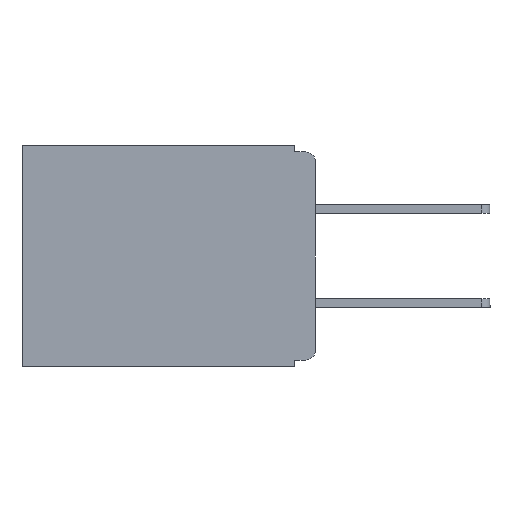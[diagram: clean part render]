
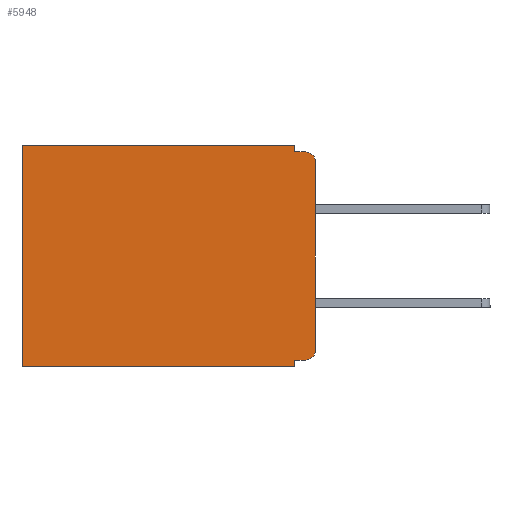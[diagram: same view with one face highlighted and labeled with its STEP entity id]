
A CAD part, left-side view. The second image highlights one B-rep face of the part: STEP entity #5948.
In plain terms, the highlighted planar face has unit normal (-1, 0, 0).
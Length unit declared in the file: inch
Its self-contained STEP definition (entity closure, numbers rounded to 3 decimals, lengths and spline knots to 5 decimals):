
#45 = DIRECTION ( 'NONE',  ( 0., 0., -1. ) ) ;
#48 = EDGE_CURVE ( 'NONE', #10251, #4668, #8956, .T. ) ;
#84 = ORIENTED_EDGE ( 'NONE', *, *, #4038, .F. ) ;
#166 = ORIENTED_EDGE ( 'NONE', *, *, #9254, .T. ) ;
#447 = CARTESIAN_POINT ( 'NONE',  ( 0.3, 0.437, 0. ) ) ;
#504 = AXIS2_PLACEMENT_3D ( 'NONE', #6257, #778, #7069 ) ;
#517 = FACE_OUTER_BOUND ( 'NONE', #5167, .T. ) ;
#527 = ORIENTED_EDGE ( 'NONE', *, *, #8979, .F. ) ;
#778 = DIRECTION ( 'NONE',  ( -1., 0., 0. ) ) ;
#1246 = DIRECTION ( 'NONE',  ( 0., 1., 0. ) ) ;
#1308 = VERTEX_POINT ( 'NONE', #2556 ) ;
#1347 = CARTESIAN_POINT ( 'NONE',  ( 0.3, 0.015, -0.32 ) ) ;
#1393 = EDGE_CURVE ( 'NONE', #7109, #4877, #10138, .T. ) ;
#1486 = ORIENTED_EDGE ( 'NONE', *, *, #9015, .T. ) ;
#1816 = CARTESIAN_POINT ( 'NONE',  ( 0.3, 0., 0. ) ) ;
#1908 = CIRCLE ( 'NONE', #504, 0.015 ) ;
#2293 = VECTOR ( 'NONE', #5901, 39.37008 ) ;
#2328 = VERTEX_POINT ( 'NONE', #2756 ) ;
#2369 = VECTOR ( 'NONE', #7701, 39.37008 ) ;
#2556 = CARTESIAN_POINT ( 'NONE',  ( 0.3, 0.031, 0. ) ) ;
#2640 = AXIS2_PLACEMENT_3D ( 'NONE', #8299, #3280, #9024 ) ;
#2756 = CARTESIAN_POINT ( 'NONE',  ( 0.3, 0., -0.305 ) ) ;
#2827 = CARTESIAN_POINT ( 'NONE',  ( 0.3, 0.031, -0.32 ) ) ;
#3158 = CARTESIAN_POINT ( 'NONE',  ( 0.3, 0.031, -0.01 ) ) ;
#3280 = DIRECTION ( 'NONE',  ( -1., 0., 0. ) ) ;
#3323 = ORIENTED_EDGE ( 'NONE', *, *, #4659, .F. ) ;
#3434 = VERTEX_POINT ( 'NONE', #7108 ) ;
#3582 = EDGE_CURVE ( 'NONE', #1308, #7109, #7062, .T. ) ;
#3742 = LINE ( 'NONE', #5969, #7959 ) ;
#3849 = VECTOR ( 'NONE', #45, 39.37008 ) ;
#4038 = EDGE_CURVE ( 'NONE', #4668, #4877, #8539, .T. ) ;
#4199 = VECTOR ( 'NONE', #10359, 39.37008 ) ;
#4332 = CARTESIAN_POINT ( 'NONE',  ( 0.3, 0., -0.33 ) ) ;
#4659 = EDGE_CURVE ( 'NONE', #1308, #5232, #3742, .T. ) ;
#4668 = VERTEX_POINT ( 'NONE', #5584 ) ;
#4790 = LINE ( 'NONE', #4332, #2369 ) ;
#4877 = VERTEX_POINT ( 'NONE', #5928 ) ;
#5167 = EDGE_LOOP ( 'NONE', ( #9774, #1486, #5932, #3323, #10086, #9341, #84, #9676, #527, #166 ) ) ;
#5197 = CARTESIAN_POINT ( 'NONE',  ( 0.3, 0.437, -0.33 ) ) ;
#5232 = VERTEX_POINT ( 'NONE', #3158 ) ;
#5358 = PLANE ( 'NONE',  #9312 ) ;
#5584 = CARTESIAN_POINT ( 'NONE',  ( 0.3, 0.031, -0.33 ) ) ;
#5602 = DIRECTION ( 'NONE',  ( 0., 0., -1. ) ) ;
#5901 = DIRECTION ( 'NONE',  ( 0., 0., -1. ) ) ;
#5928 = CARTESIAN_POINT ( 'NONE',  ( 0.3, 0.437, -0.33 ) ) ;
#5932 = ORIENTED_EDGE ( 'NONE', *, *, #8671, .F. ) ;
#5948 = ADVANCED_FACE ( 'NONE', ( #517 ), #5358, .F. ) ;
#5969 = CARTESIAN_POINT ( 'NONE',  ( 0.3, 0.031, 0. ) ) ;
#6257 = CARTESIAN_POINT ( 'NONE',  ( 0.3, 0.015, -0.305 ) ) ;
#6671 = VERTEX_POINT ( 'NONE', #8839 ) ;
#6814 = VECTOR ( 'NONE', #1246, 39.37008 ) ;
#6941 = LINE ( 'NONE', #9369, #10513 ) ;
#6987 = CARTESIAN_POINT ( 'NONE',  ( 0.3, 0., -0.33 ) ) ;
#7062 = LINE ( 'NONE', #1816, #6814 ) ;
#7069 = DIRECTION ( 'NONE',  ( 0., 0., -1. ) ) ;
#7108 = CARTESIAN_POINT ( 'NONE',  ( 0.3, 0.015, -0.01 ) ) ;
#7109 = VERTEX_POINT ( 'NONE', #447 ) ;
#7701 = DIRECTION ( 'NONE',  ( 0., 0., -1. ) ) ;
#7798 = CARTESIAN_POINT ( 'NONE',  ( 0.3, 0.031, -0.33 ) ) ;
#7888 = DIRECTION ( 'NONE',  ( 0., -1., 0. ) ) ;
#7959 = VECTOR ( 'NONE', #5602, 39.37008 ) ;
#8299 = CARTESIAN_POINT ( 'NONE',  ( 0.3, 0.015, -0.025 ) ) ;
#8457 = EDGE_CURVE ( 'NONE', #6671, #2328, #4790, .T. ) ;
#8539 = LINE ( 'NONE', #6987, #9968 ) ;
#8547 = LINE ( 'NONE', #9684, #4199 ) ;
#8671 = EDGE_CURVE ( 'NONE', #5232, #3434, #6941, .T. ) ;
#8839 = CARTESIAN_POINT ( 'NONE',  ( 0.3, 0., -0.025 ) ) ;
#8956 = LINE ( 'NONE', #7798, #2293 ) ;
#8979 = EDGE_CURVE ( 'NONE', #9745, #10251, #8547, .T. ) ;
#9015 = EDGE_CURVE ( 'NONE', #6671, #3434, #10182, .T. ) ;
#9024 = DIRECTION ( 'NONE',  ( 0., 0., -1. ) ) ;
#9098 = DIRECTION ( 'NONE',  ( 0., 1., 0. ) ) ;
#9254 = EDGE_CURVE ( 'NONE', #9745, #2328, #1908, .T. ) ;
#9312 = AXIS2_PLACEMENT_3D ( 'NONE', #10430, #9346, #9376 ) ;
#9341 = ORIENTED_EDGE ( 'NONE', *, *, #1393, .T. ) ;
#9346 = DIRECTION ( 'NONE',  ( 1., 0., 0. ) ) ;
#9369 = CARTESIAN_POINT ( 'NONE',  ( 0.3, 0., -0.01 ) ) ;
#9376 = DIRECTION ( 'NONE',  ( 0., 0., -1. ) ) ;
#9676 = ORIENTED_EDGE ( 'NONE', *, *, #48, .F. ) ;
#9684 = CARTESIAN_POINT ( 'NONE',  ( 0.3, 0., -0.32 ) ) ;
#9745 = VERTEX_POINT ( 'NONE', #1347 ) ;
#9774 = ORIENTED_EDGE ( 'NONE', *, *, #8457, .F. ) ;
#9968 = VECTOR ( 'NONE', #9098, 39.37008 ) ;
#10086 = ORIENTED_EDGE ( 'NONE', *, *, #3582, .T. ) ;
#10138 = LINE ( 'NONE', #5197, #3849 ) ;
#10182 = CIRCLE ( 'NONE', #2640, 0.015 ) ;
#10251 = VERTEX_POINT ( 'NONE', #2827 ) ;
#10359 = DIRECTION ( 'NONE',  ( 0., 1., 0. ) ) ;
#10430 = CARTESIAN_POINT ( 'NONE',  ( 0.3, 0., -0.33 ) ) ;
#10513 = VECTOR ( 'NONE', #7888, 39.37008 ) ;
